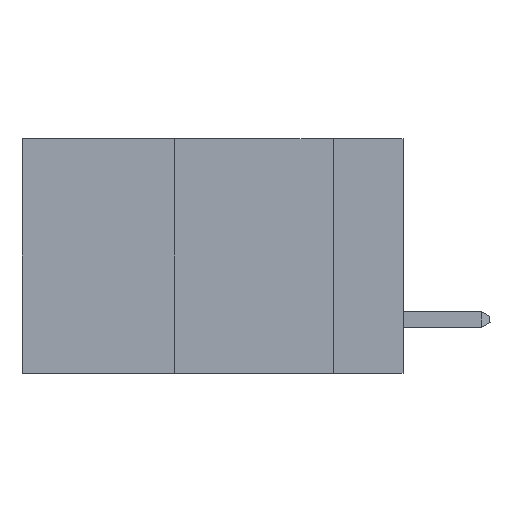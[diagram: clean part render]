
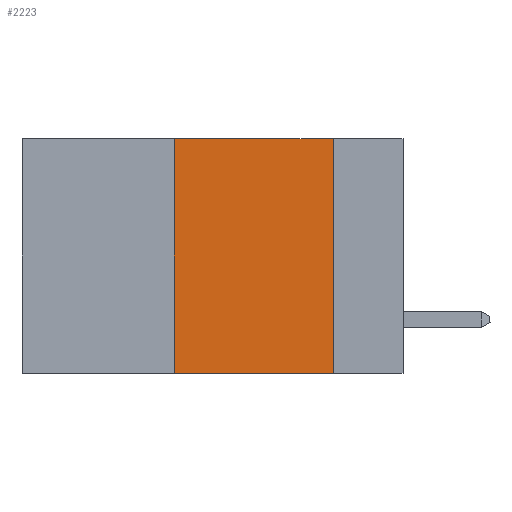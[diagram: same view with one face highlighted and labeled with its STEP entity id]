
A CAD part, left-side view. The second image highlights one B-rep face of the part: STEP entity #2223.
In plain terms, the highlighted planar face has unit normal (-1, 0, 0).
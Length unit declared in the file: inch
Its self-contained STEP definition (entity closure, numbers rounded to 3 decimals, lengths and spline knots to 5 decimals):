
#207 = ORIENTED_EDGE ( 'NONE', *, *, #410, .F. ) ;
#273 = ORIENTED_EDGE ( 'NONE', *, *, #1782, .F. ) ;
#410 = EDGE_CURVE ( 'NONE', #522, #4971, #3951, .T. ) ;
#501 = EDGE_CURVE ( 'NONE', #7798, #522, #5395, .T. ) ;
#522 = VERTEX_POINT ( 'NONE', #3989 ) ;
#779 = DIRECTION ( 'NONE',  ( 0., -1., 0. ) ) ;
#940 = DIRECTION ( 'NONE',  ( 0., 0., -1. ) ) ;
#1729 = VECTOR ( 'NONE', #2521, 39.37008 ) ;
#1782 = EDGE_CURVE ( 'NONE', #4971, #9597, #1865, .T. ) ;
#1865 = LINE ( 'NONE', #8695, #6953 ) ;
#2166 = AXIS2_PLACEMENT_3D ( 'NONE', #9109, #7159, #940 ) ;
#2223 = ADVANCED_FACE ( 'NONE', ( #9184 ), #11304, .F. ) ;
#2521 = DIRECTION ( 'NONE',  ( 0., -1., 0. ) ) ;
#2615 = CARTESIAN_POINT ( 'NONE',  ( 0., 0.36, -0.37 ) ) ;
#3951 = LINE ( 'NONE', #7597, #1729 ) ;
#3989 = CARTESIAN_POINT ( 'NONE',  ( 0., 0.36, 0. ) ) ;
#4391 = DIRECTION ( 'NONE',  ( 0., 0., -1. ) ) ;
#4846 = CARTESIAN_POINT ( 'NONE',  ( 0., 0.11, 0. ) ) ;
#4971 = VERTEX_POINT ( 'NONE', #4846 ) ;
#5097 = DIRECTION ( 'NONE',  ( 0., 0., 1. ) ) ;
#5255 = LINE ( 'NONE', #6762, #6046 ) ;
#5395 = LINE ( 'NONE', #11942, #11454 ) ;
#6046 = VECTOR ( 'NONE', #779, 39.37008 ) ;
#6107 = ORIENTED_EDGE ( 'NONE', *, *, #501, .F. ) ;
#6762 = CARTESIAN_POINT ( 'NONE',  ( 0., 0.6, -0.37 ) ) ;
#6953 = VECTOR ( 'NONE', #4391, 39.37008 ) ;
#7159 = DIRECTION ( 'NONE',  ( 1., 0., 0. ) ) ;
#7597 = CARTESIAN_POINT ( 'NONE',  ( 0., 0.6, 0. ) ) ;
#7798 = VERTEX_POINT ( 'NONE', #2615 ) ;
#8695 = CARTESIAN_POINT ( 'NONE',  ( 0., 0.11, 0. ) ) ;
#9098 = EDGE_CURVE ( 'NONE', #7798, #9597, #5255, .T. ) ;
#9109 = CARTESIAN_POINT ( 'NONE',  ( 0., 0.6, 0. ) ) ;
#9184 = FACE_OUTER_BOUND ( 'NONE', #9562, .T. ) ;
#9562 = EDGE_LOOP ( 'NONE', ( #273, #207, #6107, #12907 ) ) ;
#9597 = VERTEX_POINT ( 'NONE', #11002 ) ;
#11002 = CARTESIAN_POINT ( 'NONE',  ( 0., 0.11, -0.37 ) ) ;
#11304 = PLANE ( 'NONE',  #2166 ) ;
#11454 = VECTOR ( 'NONE', #5097, 39.37008 ) ;
#11942 = CARTESIAN_POINT ( 'NONE',  ( 0., 0.36, 0. ) ) ;
#12907 = ORIENTED_EDGE ( 'NONE', *, *, #9098, .T. ) ;
